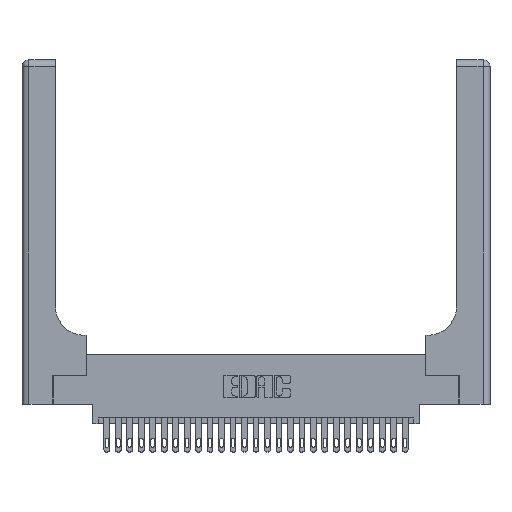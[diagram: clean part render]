
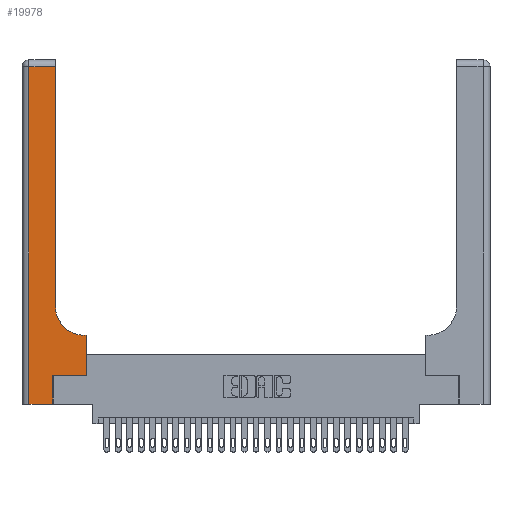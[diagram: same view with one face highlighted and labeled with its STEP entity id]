
A CAD part, top view. The second image highlights one B-rep face of the part: STEP entity #19978.
In plain terms, the highlighted planar face has unit normal (0, 0, 1).
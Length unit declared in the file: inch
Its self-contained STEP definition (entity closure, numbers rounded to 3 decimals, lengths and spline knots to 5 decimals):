
#457 = EDGE_LOOP ( 'NONE', ( #8352, #816, #15032, #26891, #28223, #24938, #7065, #15117, #23639 ) ) ;
#816 = ORIENTED_EDGE ( 'NONE', *, *, #12121, .T. ) ;
#1899 = CARTESIAN_POINT ( 'NONE',  ( 0.2915, 0.6, 0.37 ) ) ;
#1990 = VERTEX_POINT ( 'NONE', #2211 ) ;
#2117 = VECTOR ( 'NONE', #21099, 39.37008 ) ;
#2211 = CARTESIAN_POINT ( 'NONE',  ( 0.2915, 0.85, 0.37 ) ) ;
#2371 = CARTESIAN_POINT ( 'NONE',  ( 0.5415, 0.6, 0.37 ) ) ;
#2567 = EDGE_CURVE ( 'NONE', #4498, #17430, #5242, .T. ) ;
#3004 = DIRECTION ( 'NONE',  ( -1., 0., 0. ) ) ;
#3237 = EDGE_CURVE ( 'NONE', #24646, #17680, #14497, .T. ) ;
#3569 = FACE_OUTER_BOUND ( 'NONE', #457, .T. ) ;
#3652 = CIRCLE ( 'NONE', #15299, 0.25 ) ;
#4437 = DIRECTION ( 'NONE',  ( 0., -1., 0. ) ) ;
#4498 = VERTEX_POINT ( 'NONE', #8119 ) ;
#5242 = LINE ( 'NONE', #13189, #18613 ) ;
#5404 = EDGE_CURVE ( 'NONE', #25199, #25395, #12357, .T. ) ;
#6191 = DIRECTION ( 'NONE',  ( 1., 0., 0. ) ) ;
#7065 = ORIENTED_EDGE ( 'NONE', *, *, #19501, .T. ) ;
#7271 = CARTESIAN_POINT ( 'NONE',  ( 0.06, 0., 0.37 ) ) ;
#7617 = LINE ( 'NONE', #27760, #2117 ) ;
#8118 = VECTOR ( 'NONE', #6191, 39.37008 ) ;
#8119 = CARTESIAN_POINT ( 'NONE',  ( 0.06, 2.94, 0.37 ) ) ;
#8276 = CARTESIAN_POINT ( 'NONE',  ( 0.2915, 2.94, 0.37 ) ) ;
#8352 = ORIENTED_EDGE ( 'NONE', *, *, #9267, .T. ) ;
#8518 = AXIS2_PLACEMENT_3D ( 'NONE', #12044, #25010, #3004 ) ;
#8890 = EDGE_CURVE ( 'NONE', #25395, #18561, #12226, .T. ) ;
#9267 = EDGE_CURVE ( 'NONE', #1990, #17259, #26635, .T. ) ;
#9349 = CARTESIAN_POINT ( 'NONE',  ( 0.269, 0.25, 0.37 ) ) ;
#10100 = DIRECTION ( 'NONE',  ( 1., 0., 0. ) ) ;
#10355 = DIRECTION ( 'NONE',  ( 0., 1., 0. ) ) ;
#10741 = CARTESIAN_POINT ( 'NONE',  ( 0.5585, 0.25, 0.37 ) ) ;
#11493 = LINE ( 'NONE', #10741, #22827 ) ;
#12044 = CARTESIAN_POINT ( 'NONE',  ( 0., 3., 0.37 ) ) ;
#12121 = EDGE_CURVE ( 'NONE', #17259, #4498, #7617, .T. ) ;
#12211 = CARTESIAN_POINT ( 'NONE',  ( 0.5415, 0.85, 0.37 ) ) ;
#12226 = LINE ( 'NONE', #26298, #8118 ) ;
#12357 = LINE ( 'NONE', #14750, #16800 ) ;
#13189 = CARTESIAN_POINT ( 'NONE',  ( 0.06, 3., 0.37 ) ) ;
#13212 = DIRECTION ( 'NONE',  ( 0., 1., 0. ) ) ;
#13893 = DIRECTION ( 'NONE',  ( 1., 0., 0. ) ) ;
#14497 = LINE ( 'NONE', #1899, #21696 ) ;
#14750 = CARTESIAN_POINT ( 'NONE',  ( 0.269, 0., 0.37 ) ) ;
#15032 = ORIENTED_EDGE ( 'NONE', *, *, #2567, .T. ) ;
#15117 = ORIENTED_EDGE ( 'NONE', *, *, #3237, .T. ) ;
#15123 = DIRECTION ( 'NONE',  ( -1., 0., 0. ) ) ;
#15299 = AXIS2_PLACEMENT_3D ( 'NONE', #12211, #27573, #10100 ) ;
#16767 = DIRECTION ( 'NONE',  ( 0., 1., 0. ) ) ;
#16800 = VECTOR ( 'NONE', #13212, 39.37008 ) ;
#17259 = VERTEX_POINT ( 'NONE', #8276 ) ;
#17430 = VERTEX_POINT ( 'NONE', #7271 ) ;
#17680 = VERTEX_POINT ( 'NONE', #2371 ) ;
#18035 = CARTESIAN_POINT ( 'NONE',  ( 0.2915, 3., 0.37 ) ) ;
#18561 = VERTEX_POINT ( 'NONE', #25176 ) ;
#18613 = VECTOR ( 'NONE', #4437, 39.37008 ) ;
#18647 = EDGE_CURVE ( 'NONE', #17680, #1990, #3652, .T. ) ;
#18699 = LINE ( 'NONE', #27154, #24552 ) ;
#19193 = EDGE_CURVE ( 'NONE', #17430, #25199, #18699, .T. ) ;
#19501 = EDGE_CURVE ( 'NONE', #18561, #24646, #11493, .T. ) ;
#19537 = CARTESIAN_POINT ( 'NONE',  ( 0.269, 0., 0.37 ) ) ;
#19978 = ADVANCED_FACE ( 'NONE', ( #3569 ), #27119, .F. ) ;
#21099 = DIRECTION ( 'NONE',  ( -1., 0., 0. ) ) ;
#21696 = VECTOR ( 'NONE', #15123, 39.37008 ) ;
#22827 = VECTOR ( 'NONE', #10355, 39.37008 ) ;
#23639 = ORIENTED_EDGE ( 'NONE', *, *, #18647, .T. ) ;
#24552 = VECTOR ( 'NONE', #13893, 39.37008 ) ;
#24646 = VERTEX_POINT ( 'NONE', #25964 ) ;
#24938 = ORIENTED_EDGE ( 'NONE', *, *, #8890, .T. ) ;
#25010 = DIRECTION ( 'NONE',  ( 0., 0., -1. ) ) ;
#25176 = CARTESIAN_POINT ( 'NONE',  ( 0.5585, 0.25, 0.37 ) ) ;
#25199 = VERTEX_POINT ( 'NONE', #19537 ) ;
#25271 = VECTOR ( 'NONE', #16767, 39.37008 ) ;
#25395 = VERTEX_POINT ( 'NONE', #9349 ) ;
#25964 = CARTESIAN_POINT ( 'NONE',  ( 0.5585, 0.6, 0.37 ) ) ;
#26298 = CARTESIAN_POINT ( 'NONE',  ( 0.269, 0.25, 0.37 ) ) ;
#26635 = LINE ( 'NONE', #18035, #25271 ) ;
#26891 = ORIENTED_EDGE ( 'NONE', *, *, #19193, .T. ) ;
#27119 = PLANE ( 'NONE',  #8518 ) ;
#27154 = CARTESIAN_POINT ( 'NONE',  ( 0., 0., 0.37 ) ) ;
#27573 = DIRECTION ( 'NONE',  ( 0., 0., -1. ) ) ;
#27760 = CARTESIAN_POINT ( 'NONE',  ( 0., 2.94, 0.37 ) ) ;
#28223 = ORIENTED_EDGE ( 'NONE', *, *, #5404, .T. ) ;
